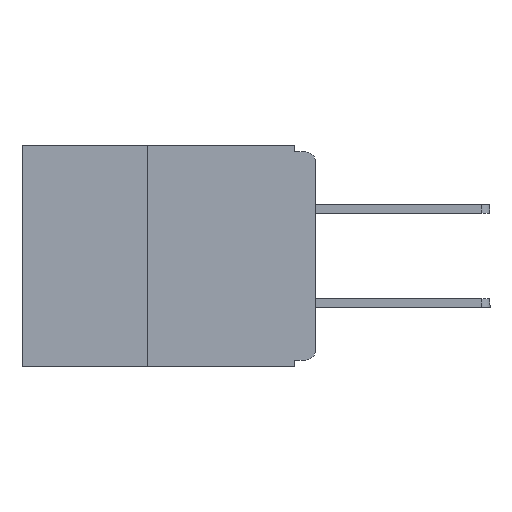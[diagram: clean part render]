
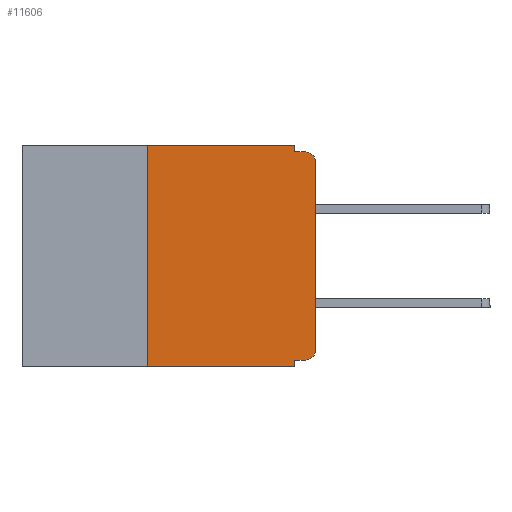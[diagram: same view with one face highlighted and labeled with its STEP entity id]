
A CAD part, left-side view. The second image highlights one B-rep face of the part: STEP entity #11606.
In plain terms, the highlighted planar face has unit normal (-1, 0, 0).
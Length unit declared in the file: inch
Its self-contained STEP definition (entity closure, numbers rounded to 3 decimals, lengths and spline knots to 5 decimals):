
#165 = VERTEX_POINT ( 'NONE', #16352 ) ;
#376 = EDGE_CURVE ( 'NONE', #17158, #3627, #15402, .T. ) ;
#411 = CARTESIAN_POINT ( 'NONE',  ( 0., 0.031, 0. ) ) ;
#858 = EDGE_CURVE ( 'NONE', #18260, #17158, #7855, .T. ) ;
#872 = DIRECTION ( 'NONE',  ( 0., 0., -1. ) ) ;
#889 = DIRECTION ( 'NONE',  ( -1., 0., 0. ) ) ;
#895 = CARTESIAN_POINT ( 'NONE',  ( 0., 0.015, -0.025 ) ) ;
#965 = VERTEX_POINT ( 'NONE', #13876 ) ;
#1142 = LINE ( 'NONE', #14392, #13484 ) ;
#1186 = LINE ( 'NONE', #12926, #4434 ) ;
#1486 = ORIENTED_EDGE ( 'NONE', *, *, #18355, .T. ) ;
#1760 = AXIS2_PLACEMENT_3D ( 'NONE', #2011, #12786, #3612 ) ;
#1790 = ORIENTED_EDGE ( 'NONE', *, *, #15382, .F. ) ;
#2011 = CARTESIAN_POINT ( 'NONE',  ( 0., 0.015, -0.305 ) ) ;
#2797 = VERTEX_POINT ( 'NONE', #4067 ) ;
#2883 = CIRCLE ( 'NONE', #1760, 0.015 ) ;
#3311 = VECTOR ( 'NONE', #16138, 39.37008 ) ;
#3612 = DIRECTION ( 'NONE',  ( 0., 0., -1. ) ) ;
#3627 = VERTEX_POINT ( 'NONE', #11399 ) ;
#3657 = VECTOR ( 'NONE', #14431, 39.37008 ) ;
#3669 = PLANE ( 'NONE',  #7882 ) ;
#4067 = CARTESIAN_POINT ( 'NONE',  ( 0., 0., -0.025 ) ) ;
#4209 = VERTEX_POINT ( 'NONE', #411 ) ;
#4434 = VECTOR ( 'NONE', #12657, 39.37008 ) ;
#4505 = ORIENTED_EDGE ( 'NONE', *, *, #376, .F. ) ;
#4670 = EDGE_LOOP ( 'NONE', ( #7081, #10672, #15524, #8438, #1790, #12177, #14008, #4505, #13783, #1486 ) ) ;
#4675 = EDGE_CURVE ( 'NONE', #6305, #3627, #1186, .T. ) ;
#4905 = CARTESIAN_POINT ( 'NONE',  ( 0., 0., -0.305 ) ) ;
#5314 = CIRCLE ( 'NONE', #15610, 0.015 ) ;
#5405 = LINE ( 'NONE', #15627, #17042 ) ;
#5601 = EDGE_CURVE ( 'NONE', #15080, #2797, #1142, .T. ) ;
#6305 = VERTEX_POINT ( 'NONE', #8137 ) ;
#6822 = DIRECTION ( 'NONE',  ( 1., 0., 0. ) ) ;
#6961 = EDGE_CURVE ( 'NONE', #2797, #9276, #5314, .T. ) ;
#7081 = ORIENTED_EDGE ( 'NONE', *, *, #5601, .T. ) ;
#7337 = CARTESIAN_POINT ( 'NONE',  ( 0., 0.031, -0.33 ) ) ;
#7500 = LINE ( 'NONE', #18969, #3311 ) ;
#7855 = LINE ( 'NONE', #14697, #3657 ) ;
#7882 = AXIS2_PLACEMENT_3D ( 'NONE', #15891, #6822, #17374 ) ;
#7914 = VECTOR ( 'NONE', #13262, 39.37008 ) ;
#8137 = CARTESIAN_POINT ( 'NONE',  ( 0., 0.25, -0.33 ) ) ;
#8438 = ORIENTED_EDGE ( 'NONE', *, *, #14902, .F. ) ;
#8858 = EDGE_CURVE ( 'NONE', #6305, #965, #7500, .T. ) ;
#9200 = DIRECTION ( 'NONE',  ( 0., 0., -1. ) ) ;
#9276 = VERTEX_POINT ( 'NONE', #15864 ) ;
#9612 = DIRECTION ( 'NONE',  ( 0., -1., 0. ) ) ;
#10672 = ORIENTED_EDGE ( 'NONE', *, *, #6961, .T. ) ;
#10937 = CARTESIAN_POINT ( 'NONE',  ( 0., 0.015, -0.32 ) ) ;
#11243 = CARTESIAN_POINT ( 'NONE',  ( 0., 0.031, -0.32 ) ) ;
#11368 = VECTOR ( 'NONE', #16860, 39.37008 ) ;
#11399 = CARTESIAN_POINT ( 'NONE',  ( 0., 0.031, -0.33 ) ) ;
#11606 = ADVANCED_FACE ( 'NONE', ( #19163 ), #3669, .F. ) ;
#12177 = ORIENTED_EDGE ( 'NONE', *, *, #8858, .F. ) ;
#12573 = VECTOR ( 'NONE', #9200, 39.37008 ) ;
#12657 = DIRECTION ( 'NONE',  ( 0., -1., 0. ) ) ;
#12786 = DIRECTION ( 'NONE',  ( -1., 0., 0. ) ) ;
#12926 = CARTESIAN_POINT ( 'NONE',  ( 0., 0.437, -0.33 ) ) ;
#13262 = DIRECTION ( 'NONE',  ( 0., -1., 0. ) ) ;
#13484 = VECTOR ( 'NONE', #14523, 39.37008 ) ;
#13783 = ORIENTED_EDGE ( 'NONE', *, *, #858, .F. ) ;
#13876 = CARTESIAN_POINT ( 'NONE',  ( 0., 0.25, 0. ) ) ;
#14008 = ORIENTED_EDGE ( 'NONE', *, *, #4675, .T. ) ;
#14392 = CARTESIAN_POINT ( 'NONE',  ( 0., 0., 0. ) ) ;
#14431 = DIRECTION ( 'NONE',  ( 0., 1., 0. ) ) ;
#14523 = DIRECTION ( 'NONE',  ( 0., 0., 1. ) ) ;
#14697 = CARTESIAN_POINT ( 'NONE',  ( 0., 0., -0.32 ) ) ;
#14902 = EDGE_CURVE ( 'NONE', #4209, #165, #16581, .T. ) ;
#15080 = VERTEX_POINT ( 'NONE', #4905 ) ;
#15190 = CARTESIAN_POINT ( 'NONE',  ( 0., 0.031, 0. ) ) ;
#15382 = EDGE_CURVE ( 'NONE', #965, #4209, #19711, .T. ) ;
#15402 = LINE ( 'NONE', #7337, #11368 ) ;
#15524 = ORIENTED_EDGE ( 'NONE', *, *, #16599, .F. ) ;
#15610 = AXIS2_PLACEMENT_3D ( 'NONE', #895, #889, #872 ) ;
#15627 = CARTESIAN_POINT ( 'NONE',  ( 0., 0., -0.01 ) ) ;
#15864 = CARTESIAN_POINT ( 'NONE',  ( 0., 0.015, -0.01 ) ) ;
#15891 = CARTESIAN_POINT ( 'NONE',  ( 0., 0.437, 0. ) ) ;
#16138 = DIRECTION ( 'NONE',  ( 0., 0., 1. ) ) ;
#16234 = CARTESIAN_POINT ( 'NONE',  ( 0., 0.437, 0. ) ) ;
#16352 = CARTESIAN_POINT ( 'NONE',  ( 0., 0.031, -0.01 ) ) ;
#16581 = LINE ( 'NONE', #15190, #12573 ) ;
#16599 = EDGE_CURVE ( 'NONE', #165, #9276, #5405, .T. ) ;
#16860 = DIRECTION ( 'NONE',  ( 0., 0., -1. ) ) ;
#17042 = VECTOR ( 'NONE', #9612, 39.37008 ) ;
#17158 = VERTEX_POINT ( 'NONE', #11243 ) ;
#17374 = DIRECTION ( 'NONE',  ( 0., 0., -1. ) ) ;
#18260 = VERTEX_POINT ( 'NONE', #10937 ) ;
#18355 = EDGE_CURVE ( 'NONE', #18260, #15080, #2883, .T. ) ;
#18969 = CARTESIAN_POINT ( 'NONE',  ( 0., 0.25, -0.33 ) ) ;
#19163 = FACE_OUTER_BOUND ( 'NONE', #4670, .T. ) ;
#19711 = LINE ( 'NONE', #16234, #7914 ) ;
